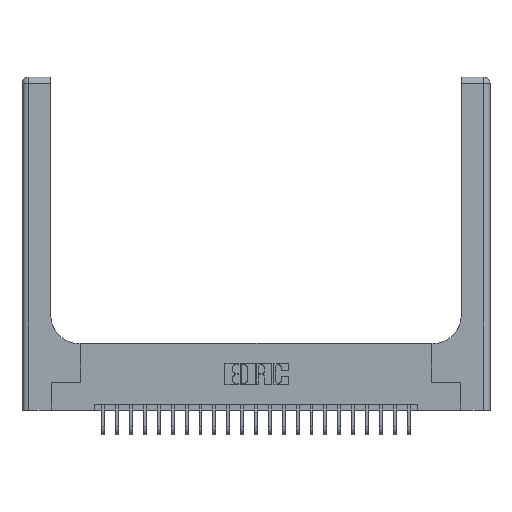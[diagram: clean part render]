
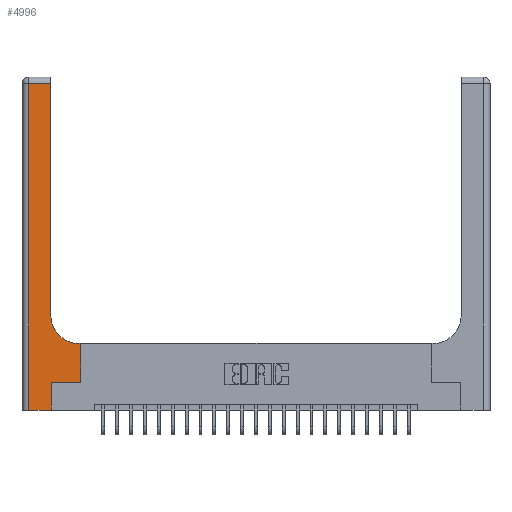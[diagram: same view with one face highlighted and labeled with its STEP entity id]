
A CAD part, top view. The second image highlights one B-rep face of the part: STEP entity #4996.
In plain terms, the highlighted planar face has unit normal (0, 0, 1).
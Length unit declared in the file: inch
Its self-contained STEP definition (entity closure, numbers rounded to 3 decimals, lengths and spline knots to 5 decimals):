
#547 = AXIS2_PLACEMENT_3D ( 'NONE', #23319, #13412, #19112 ) ;
#719 = LINE ( 'NONE', #21713, #1820 ) ;
#997 = VERTEX_POINT ( 'NONE', #6053 ) ;
#1099 = VERTEX_POINT ( 'NONE', #2882 ) ;
#1124 = CARTESIAN_POINT ( 'NONE',  ( 0.06, 2.94, 0.37 ) ) ;
#1206 = ORIENTED_EDGE ( 'NONE', *, *, #5628, .T. ) ;
#1240 = EDGE_CURVE ( 'NONE', #997, #10188, #7301, .T. ) ;
#1820 = VECTOR ( 'NONE', #12211, 39.37008 ) ;
#1987 = CARTESIAN_POINT ( 'NONE',  ( 0.265, 0.25, 0.37 ) ) ;
#2606 = DIRECTION ( 'NONE',  ( 0., 1., 0. ) ) ;
#2666 = ORIENTED_EDGE ( 'NONE', *, *, #18090, .T. ) ;
#2827 = EDGE_CURVE ( 'NONE', #22382, #21609, #11109, .T. ) ;
#2882 = CARTESIAN_POINT ( 'NONE',  ( 0.528, 0.6, 0.37 ) ) ;
#3360 = ORIENTED_EDGE ( 'NONE', *, *, #11419, .T. ) ;
#3526 = ORIENTED_EDGE ( 'NONE', *, *, #13683, .T. ) ;
#3561 = EDGE_CURVE ( 'NONE', #1099, #20913, #20779, .T. ) ;
#3884 = DIRECTION ( 'NONE',  ( 1., 0., 0. ) ) ;
#3952 = LINE ( 'NONE', #17467, #11877 ) ;
#4344 = CARTESIAN_POINT ( 'NONE',  ( 0.528, 0.25, 0.37 ) ) ;
#4881 = CARTESIAN_POINT ( 'NONE',  ( 0.265, 0., 0.37 ) ) ;
#4966 = CIRCLE ( 'NONE', #547, 0.25 ) ;
#4996 = ADVANCED_FACE ( 'NONE', ( #23574 ), #17938, .F. ) ;
#5628 = EDGE_CURVE ( 'NONE', #10030, #24925, #9450, .T. ) ;
#5662 = CARTESIAN_POINT ( 'NONE',  ( 0., 0., 0.37 ) ) ;
#6053 = CARTESIAN_POINT ( 'NONE',  ( 0.265, 0.25, 0.37 ) ) ;
#6328 = CARTESIAN_POINT ( 'NONE',  ( 0., 3., 0.37 ) ) ;
#6830 = AXIS2_PLACEMENT_3D ( 'NONE', #6328, #9871, #21768 ) ;
#7003 = DIRECTION ( 'NONE',  ( 0., 1., 0. ) ) ;
#7051 = EDGE_CURVE ( 'NONE', #10188, #1099, #9022, .T. ) ;
#7301 = LINE ( 'NONE', #1987, #15823 ) ;
#7446 = DIRECTION ( 'NONE',  ( 1., 0., 0. ) ) ;
#8146 = CARTESIAN_POINT ( 'NONE',  ( 0.26, 2.94, 0.37 ) ) ;
#9022 = LINE ( 'NONE', #20677, #22621 ) ;
#9450 = LINE ( 'NONE', #5662, #21655 ) ;
#9871 = DIRECTION ( 'NONE',  ( 0., 0., -1. ) ) ;
#10030 = VERTEX_POINT ( 'NONE', #16350 ) ;
#10188 = VERTEX_POINT ( 'NONE', #4344 ) ;
#10539 = ORIENTED_EDGE ( 'NONE', *, *, #12724, .T. ) ;
#11109 = LINE ( 'NONE', #24549, #11185 ) ;
#11185 = VECTOR ( 'NONE', #18671, 39.37008 ) ;
#11419 = EDGE_CURVE ( 'NONE', #20913, #12678, #4966, .T. ) ;
#11877 = VECTOR ( 'NONE', #21037, 39.37008 ) ;
#12211 = DIRECTION ( 'NONE',  ( 0., -1., 0. ) ) ;
#12678 = VERTEX_POINT ( 'NONE', #17212 ) ;
#12724 = EDGE_CURVE ( 'NONE', #12678, #22382, #3952, .T. ) ;
#13412 = DIRECTION ( 'NONE',  ( 0., 0., -1. ) ) ;
#13531 = CARTESIAN_POINT ( 'NONE',  ( 0.26, 0.6, 0.37 ) ) ;
#13683 = EDGE_CURVE ( 'NONE', #21609, #10030, #719, .T. ) ;
#14143 = CARTESIAN_POINT ( 'NONE',  ( 0.265, 0., 0.37 ) ) ;
#15134 = EDGE_LOOP ( 'NONE', ( #10539, #24427, #3526, #1206, #2666, #20912, #18067, #15802, #3360 ) ) ;
#15449 = DIRECTION ( 'NONE',  ( -1., 0., 0. ) ) ;
#15802 = ORIENTED_EDGE ( 'NONE', *, *, #3561, .T. ) ;
#15823 = VECTOR ( 'NONE', #3884, 39.37008 ) ;
#16115 = LINE ( 'NONE', #4881, #24613 ) ;
#16350 = CARTESIAN_POINT ( 'NONE',  ( 0.06, 0., 0.37 ) ) ;
#17212 = CARTESIAN_POINT ( 'NONE',  ( 0.26, 0.85, 0.37 ) ) ;
#17467 = CARTESIAN_POINT ( 'NONE',  ( 0.26, 3., 0.37 ) ) ;
#17938 = PLANE ( 'NONE',  #6830 ) ;
#18067 = ORIENTED_EDGE ( 'NONE', *, *, #7051, .T. ) ;
#18090 = EDGE_CURVE ( 'NONE', #24925, #997, #16115, .T. ) ;
#18671 = DIRECTION ( 'NONE',  ( -1., 0., 0. ) ) ;
#19112 = DIRECTION ( 'NONE',  ( 1., 0., 0. ) ) ;
#20677 = CARTESIAN_POINT ( 'NONE',  ( 0.528, 0.25, 0.37 ) ) ;
#20779 = LINE ( 'NONE', #13531, #22633 ) ;
#20912 = ORIENTED_EDGE ( 'NONE', *, *, #1240, .T. ) ;
#20913 = VERTEX_POINT ( 'NONE', #24643 ) ;
#21037 = DIRECTION ( 'NONE',  ( 0., 1., 0. ) ) ;
#21609 = VERTEX_POINT ( 'NONE', #1124 ) ;
#21655 = VECTOR ( 'NONE', #7446, 39.37008 ) ;
#21713 = CARTESIAN_POINT ( 'NONE',  ( 0.06, 3., 0.37 ) ) ;
#21768 = DIRECTION ( 'NONE',  ( -1., 0., 0. ) ) ;
#22382 = VERTEX_POINT ( 'NONE', #8146 ) ;
#22621 = VECTOR ( 'NONE', #7003, 39.37008 ) ;
#22633 = VECTOR ( 'NONE', #15449, 39.37008 ) ;
#23319 = CARTESIAN_POINT ( 'NONE',  ( 0.51, 0.85, 0.37 ) ) ;
#23574 = FACE_OUTER_BOUND ( 'NONE', #15134, .T. ) ;
#24427 = ORIENTED_EDGE ( 'NONE', *, *, #2827, .T. ) ;
#24549 = CARTESIAN_POINT ( 'NONE',  ( 0., 2.94, 0.37 ) ) ;
#24613 = VECTOR ( 'NONE', #2606, 39.37008 ) ;
#24643 = CARTESIAN_POINT ( 'NONE',  ( 0.51, 0.6, 0.37 ) ) ;
#24925 = VERTEX_POINT ( 'NONE', #14143 ) ;
